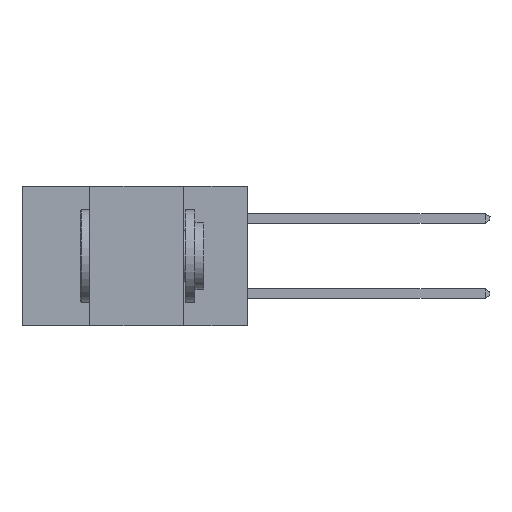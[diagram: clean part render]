
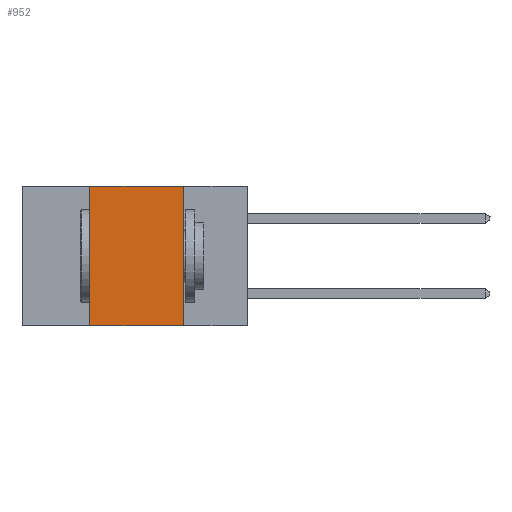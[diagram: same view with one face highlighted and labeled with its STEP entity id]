
A CAD part, left-side view. The second image highlights one B-rep face of the part: STEP entity #952.
In plain terms, the highlighted planar face has unit normal (-1, 0, 0).
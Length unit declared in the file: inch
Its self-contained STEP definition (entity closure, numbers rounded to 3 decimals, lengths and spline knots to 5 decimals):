
#209 = DIRECTION ( 'NONE',  ( 0., -1., 0. ) ) ;
#457 = DIRECTION ( 'NONE',  ( 0., 0., -1. ) ) ;
#521 = ORIENTED_EDGE ( 'NONE', *, *, #10210, .T. ) ;
#898 = DIRECTION ( 'NONE',  ( 1., 0., 0. ) ) ;
#952 = ADVANCED_FACE ( 'NONE', ( #15302 ), #8746, .F. ) ;
#1173 = VECTOR ( 'NONE', #4132, 39.37008 ) ;
#2210 = EDGE_CURVE ( 'NONE', #11730, #5004, #14096, .T. ) ;
#3070 = ORIENTED_EDGE ( 'NONE', *, *, #14282, .F. ) ;
#3879 = CARTESIAN_POINT ( 'NONE',  ( 0., 0.6, 0. ) ) ;
#4132 = DIRECTION ( 'NONE',  ( 0., -1., 0. ) ) ;
#5004 = VERTEX_POINT ( 'NONE', #8265 ) ;
#5032 = CARTESIAN_POINT ( 'NONE',  ( 0., 0.42, -0.37 ) ) ;
#5727 = VECTOR ( 'NONE', #209, 39.37008 ) ;
#6157 = DIRECTION ( 'NONE',  ( 0., 0., -1. ) ) ;
#6172 = CARTESIAN_POINT ( 'NONE',  ( 0., 0.17, 0. ) ) ;
#6381 = ORIENTED_EDGE ( 'NONE', *, *, #14635, .F. ) ;
#7358 = CARTESIAN_POINT ( 'NONE',  ( 0., 0.17, -0.37 ) ) ;
#8062 = LINE ( 'NONE', #11992, #5727 ) ;
#8265 = CARTESIAN_POINT ( 'NONE',  ( 0., 0.42, 0. ) ) ;
#8746 = PLANE ( 'NONE',  #13959 ) ;
#8868 = VECTOR ( 'NONE', #457, 39.37008 ) ;
#9395 = CARTESIAN_POINT ( 'NONE',  ( 0., 0.17, -0.37 ) ) ;
#9582 = LINE ( 'NONE', #7358, #8868 ) ;
#9876 = VERTEX_POINT ( 'NONE', #6172 ) ;
#10210 = EDGE_CURVE ( 'NONE', #11730, #14530, #8062, .T. ) ;
#10448 = LINE ( 'NONE', #3879, #1173 ) ;
#11730 = VERTEX_POINT ( 'NONE', #15213 ) ;
#11801 = ORIENTED_EDGE ( 'NONE', *, *, #2210, .F. ) ;
#11992 = CARTESIAN_POINT ( 'NONE',  ( 0., 0.6, -0.37 ) ) ;
#12713 = CARTESIAN_POINT ( 'NONE',  ( 0., 0.6, 0. ) ) ;
#12717 = DIRECTION ( 'NONE',  ( 0., 0., 1. ) ) ;
#13407 = EDGE_LOOP ( 'NONE', ( #3070, #6381, #11801, #521 ) ) ;
#13959 = AXIS2_PLACEMENT_3D ( 'NONE', #12713, #898, #6157 ) ;
#14096 = LINE ( 'NONE', #5032, #14973 ) ;
#14282 = EDGE_CURVE ( 'NONE', #9876, #14530, #9582, .T. ) ;
#14530 = VERTEX_POINT ( 'NONE', #9395 ) ;
#14635 = EDGE_CURVE ( 'NONE', #5004, #9876, #10448, .T. ) ;
#14973 = VECTOR ( 'NONE', #12717, 39.37008 ) ;
#15213 = CARTESIAN_POINT ( 'NONE',  ( 0., 0.42, -0.37 ) ) ;
#15302 = FACE_OUTER_BOUND ( 'NONE', #13407, .T. ) ;
